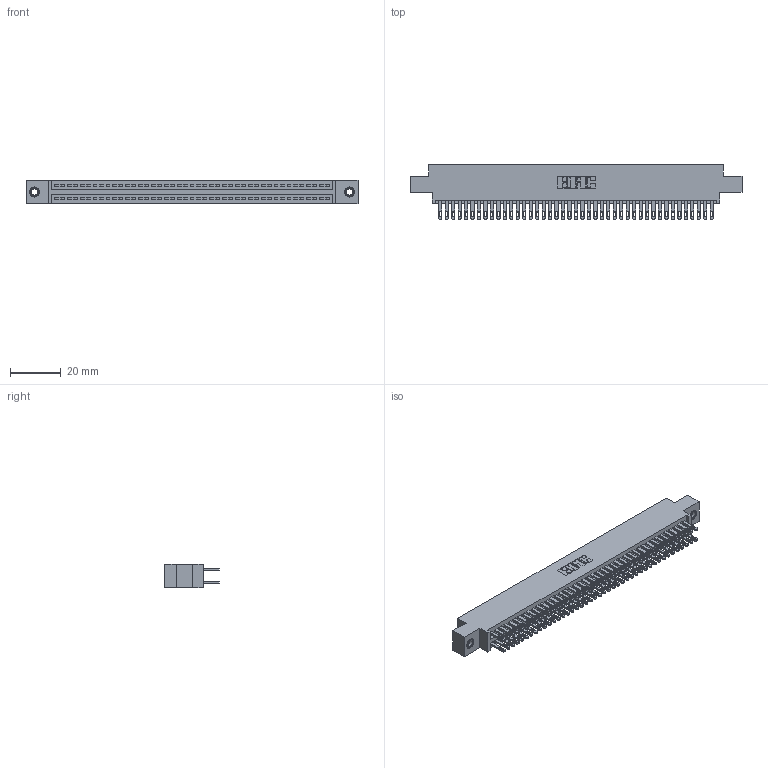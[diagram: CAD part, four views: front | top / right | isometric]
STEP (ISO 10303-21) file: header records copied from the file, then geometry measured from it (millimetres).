
FILE_DESCRIPTION (( 'STEP AP203' ), '1' );
FILE_NAME ('345-086-500-807.STEP', '2018-10-04T04:09:48', ( '' ), ( '' ), 'SwSTEP 2.0', 'SolidWorks 2016', '' );
FILE_SCHEMA (( 'CONFIG_CONTROL_DESIGN' ));
Length unit declared in the file: inch
Products named in the file (4): 345-250-001_345-250-005-103; 345-086-500-807; 345 Part_0.170 Offset - 0.156 Dia-TI; 345-292-001_345-293-100
Assembly tree (89 placements, depth 2):
  345-086-500-807
    345 Part_0.170 Offset - 0.156 Dia-TI
    345-292-001_345-293-100  x86
    345-250-001_345-250-005-103  x2
Bounding box: 130.43 x 21.51 x 9.4 mm (x, y, z)
Volume: 12815.2 mm3; surface area: 20010.9 mm2
Topology: 89 solids, 89 shells, 4146 faces, 12615 edges, 8402 vertices
Faces by surface type: plane 2438, cylinder 1692, cone 12, torus 4
Entity records: 34852 total; most frequent: CARTESIAN_POINT 5823, ORIENTED_EDGE 5750, DIRECTION 5161, EDGE_CURVE 2875, LINE 2547, VECTOR 2547, VERTEX_POINT 1912, AXIS2_PLACEMENT_3D 1307
